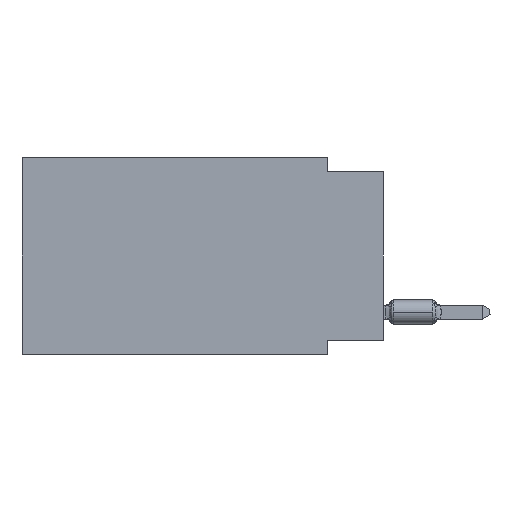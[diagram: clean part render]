
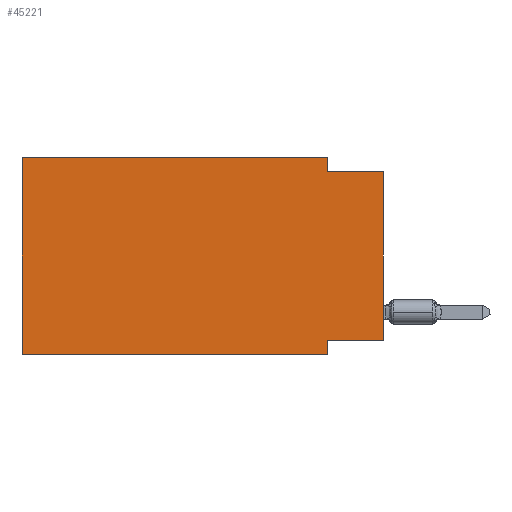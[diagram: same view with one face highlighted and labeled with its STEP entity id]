
A CAD part, left-side view. The second image highlights one B-rep face of the part: STEP entity #45221.
In plain terms, the highlighted planar face has unit normal (-1, 0, 0).
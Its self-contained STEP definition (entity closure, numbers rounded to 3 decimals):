
#304 = CARTESIAN_POINT ( 'NONE',  ( 0., 2.54, -0.635 ) ) ;
#1030 = DIRECTION ( 'NONE',  ( 0., -1., 0. ) ) ;
#5586 = VECTOR ( 'NONE', #12209, 1000. ) ;
#5741 = EDGE_CURVE ( 'NONE', #82244, #55861, #66307, .T. ) ;
#5747 = CARTESIAN_POINT ( 'NONE',  ( 0., 0., -8.255 ) ) ;
#6076 = LINE ( 'NONE', #70318, #102316 ) ;
#6174 = ORIENTED_EDGE ( 'NONE', *, *, #5741, .F. ) ;
#7044 = EDGE_LOOP ( 'NONE', ( #23532, #6174, #70614, #56650, #48169, #84348, #61116, #95149 ) ) ;
#7312 = LINE ( 'NONE', #85825, #62042 ) ;
#8358 = DIRECTION ( 'NONE',  ( 0., -1., 0. ) ) ;
#8640 = AXIS2_PLACEMENT_3D ( 'NONE', #25098, #40922, #34026 ) ;
#12209 = DIRECTION ( 'NONE',  ( 0., -1., 0. ) ) ;
#15204 = VERTEX_POINT ( 'NONE', #43294 ) ;
#23532 = ORIENTED_EDGE ( 'NONE', *, *, #32007, .T. ) ;
#24760 = EDGE_CURVE ( 'NONE', #15204, #92348, #6076, .T. ) ;
#25098 = CARTESIAN_POINT ( 'NONE',  ( 0., 16.383, 0. ) ) ;
#29383 = EDGE_CURVE ( 'NONE', #93372, #15204, #36329, .T. ) ;
#32007 = EDGE_CURVE ( 'NONE', #93372, #55861, #71392, .T. ) ;
#32778 = VECTOR ( 'NONE', #1030, 1000. ) ;
#34026 = DIRECTION ( 'NONE',  ( 0., 0., -1. ) ) ;
#34594 = EDGE_CURVE ( 'NONE', #51570, #82244, #46002, .T. ) ;
#36329 = LINE ( 'NONE', #5747, #97704 ) ;
#38459 = VECTOR ( 'NONE', #8358, 1000. ) ;
#40922 = DIRECTION ( 'NONE',  ( 1., 0., 0. ) ) ;
#41358 = CARTESIAN_POINT ( 'NONE',  ( 0., 0., -8.255 ) ) ;
#43294 = CARTESIAN_POINT ( 'NONE',  ( 0., 2.54, -8.255 ) ) ;
#43633 = VERTEX_POINT ( 'NONE', #73151 ) ;
#45221 = ADVANCED_FACE ( 'NONE', ( #97781 ), #74061, .F. ) ;
#46002 = LINE ( 'NONE', #54941, #96579 ) ;
#48169 = ORIENTED_EDGE ( 'NONE', *, *, #83519, .F. ) ;
#48936 = EDGE_CURVE ( 'NONE', #57462, #92348, #96890, .T. ) ;
#51570 = VERTEX_POINT ( 'NONE', #58215 ) ;
#54941 = CARTESIAN_POINT ( 'NONE',  ( 0., 2.54, 0. ) ) ;
#55076 = CARTESIAN_POINT ( 'NONE',  ( 0., 0., 0. ) ) ;
#55861 = VERTEX_POINT ( 'NONE', #71458 ) ;
#56650 = ORIENTED_EDGE ( 'NONE', *, *, #99320, .F. ) ;
#57462 = VERTEX_POINT ( 'NONE', #90776 ) ;
#57783 = VECTOR ( 'NONE', #87217, 1000. ) ;
#58215 = CARTESIAN_POINT ( 'NONE',  ( 0., 2.54, 0. ) ) ;
#60541 = DIRECTION ( 'NONE',  ( 0., 1., 0. ) ) ;
#61116 = ORIENTED_EDGE ( 'NONE', *, *, #24760, .F. ) ;
#62042 = VECTOR ( 'NONE', #94779, 1000. ) ;
#66307 = LINE ( 'NONE', #97421, #32778 ) ;
#69083 = CARTESIAN_POINT ( 'NONE',  ( 0., 16.383, 0. ) ) ;
#70318 = CARTESIAN_POINT ( 'NONE',  ( 0., 2.54, -8.89 ) ) ;
#70614 = ORIENTED_EDGE ( 'NONE', *, *, #34594, .F. ) ;
#71392 = LINE ( 'NONE', #55076, #57783 ) ;
#71458 = CARTESIAN_POINT ( 'NONE',  ( 0., 0., -0.635 ) ) ;
#73151 = CARTESIAN_POINT ( 'NONE',  ( 0., 16.383, 0. ) ) ;
#74061 = PLANE ( 'NONE',  #8640 ) ;
#82244 = VERTEX_POINT ( 'NONE', #304 ) ;
#83519 = EDGE_CURVE ( 'NONE', #57462, #43633, #7312, .T. ) ;
#84348 = ORIENTED_EDGE ( 'NONE', *, *, #48936, .T. ) ;
#85498 = DIRECTION ( 'NONE',  ( 0., 0., -1. ) ) ;
#85825 = CARTESIAN_POINT ( 'NONE',  ( 0., 16.383, 0. ) ) ;
#85946 = LINE ( 'NONE', #69083, #5586 ) ;
#87217 = DIRECTION ( 'NONE',  ( 0., 0., 1. ) ) ;
#90776 = CARTESIAN_POINT ( 'NONE',  ( 0., 16.383, -8.89 ) ) ;
#92348 = VERTEX_POINT ( 'NONE', #99166 ) ;
#93372 = VERTEX_POINT ( 'NONE', #41358 ) ;
#94779 = DIRECTION ( 'NONE',  ( 0., 0., 1. ) ) ;
#95149 = ORIENTED_EDGE ( 'NONE', *, *, #29383, .F. ) ;
#96579 = VECTOR ( 'NONE', #85498, 1000. ) ;
#96890 = LINE ( 'NONE', #99839, #38459 ) ;
#97421 = CARTESIAN_POINT ( 'NONE',  ( 0., 0., -0.635 ) ) ;
#97704 = VECTOR ( 'NONE', #60541, 1000. ) ;
#97781 = FACE_OUTER_BOUND ( 'NONE', #7044, .T. ) ;
#99166 = CARTESIAN_POINT ( 'NONE',  ( 0., 2.54, -8.89 ) ) ;
#99320 = EDGE_CURVE ( 'NONE', #43633, #51570, #85946, .T. ) ;
#99839 = CARTESIAN_POINT ( 'NONE',  ( 0., 16.383, -8.89 ) ) ;
#102316 = VECTOR ( 'NONE', #102473, 1000. ) ;
#102473 = DIRECTION ( 'NONE',  ( 0., 0., -1. ) ) ;
